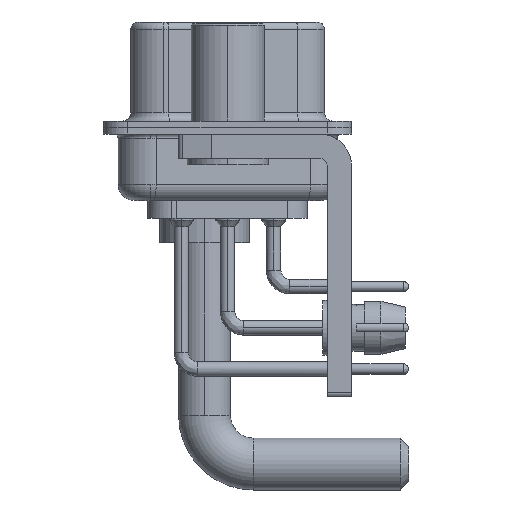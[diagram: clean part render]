
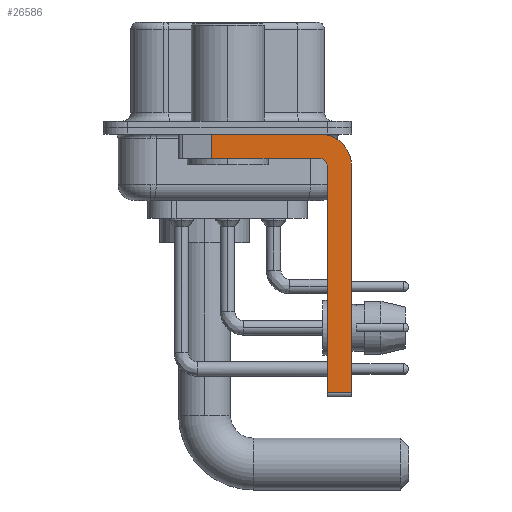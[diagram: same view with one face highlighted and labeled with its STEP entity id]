
A CAD part, left-side view. The second image highlights one B-rep face of the part: STEP entity #26586.
In plain terms, the highlighted planar face has unit normal (-1, 0, 0).
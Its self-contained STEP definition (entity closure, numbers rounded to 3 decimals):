
#164 = ORIENTED_EDGE ( 'NONE', *, *, #16579, .F. ) ;
#937 = CARTESIAN_POINT ( 'NONE',  ( -2.9, 0.978, -1.9 ) ) ;
#2447 = ORIENTED_EDGE ( 'NONE', *, *, #3373, .F. ) ;
#3217 = CARTESIAN_POINT ( 'NONE',  ( -2.9, -5.65, -2.4 ) ) ;
#3373 = EDGE_CURVE ( 'NONE', #6912, #23602, #33121, .T. ) ;
#3415 = EDGE_CURVE ( 'NONE', #27893, #8303, #26607, .T. ) ;
#3915 = AXIS2_PLACEMENT_3D ( 'NONE', #36404, #33342, #8636 ) ;
#4484 = VERTEX_POINT ( 'NONE', #37682 ) ;
#4507 = EDGE_CURVE ( 'NONE', #18690, #8303, #25046, .T. ) ;
#5152 = FACE_OUTER_BOUND ( 'NONE', #33756, .T. ) ;
#5398 = LINE ( 'NONE', #17841, #13800 ) ;
#5410 = AXIS2_PLACEMENT_3D ( 'NONE', #33012, #17060, #36479 ) ;
#5933 = AXIS2_PLACEMENT_3D ( 'NONE', #3217, #28167, #9552 ) ;
#6912 = VERTEX_POINT ( 'NONE', #35446 ) ;
#7973 = CARTESIAN_POINT ( 'NONE',  ( -2.9, -6.15, -16.35 ) ) ;
#8303 = VERTEX_POINT ( 'NONE', #12050 ) ;
#8636 = DIRECTION ( 'NONE',  ( 0., 0., -1. ) ) ;
#8646 = LINE ( 'NONE', #30895, #10267 ) ;
#9231 = ORIENTED_EDGE ( 'NONE', *, *, #22235, .F. ) ;
#9552 = DIRECTION ( 'NONE',  ( 0., 0., 1. ) ) ;
#10046 = EDGE_CURVE ( 'NONE', #30020, #6912, #37889, .T. ) ;
#10143 = ORIENTED_EDGE ( 'NONE', *, *, #3415, .T. ) ;
#10267 = VECTOR ( 'NONE', #33157, 1000. ) ;
#10851 = DIRECTION ( 'NONE',  ( 0., -1., 0. ) ) ;
#11998 = ORIENTED_EDGE ( 'NONE', *, *, #4507, .F. ) ;
#12050 = CARTESIAN_POINT ( 'NONE',  ( -2.9, -7.65, -16.35 ) ) ;
#12092 = EDGE_CURVE ( 'NONE', #27893, #30020, #5398, .T. ) ;
#12316 = CARTESIAN_POINT ( 'NONE',  ( -2.9, 0.978, -1.9 ) ) ;
#13800 = VECTOR ( 'NONE', #26881, 1000. ) ;
#13990 = LINE ( 'NONE', #937, #34609 ) ;
#16579 = EDGE_CURVE ( 'NONE', #4484, #18690, #20413, .T. ) ;
#16966 = DIRECTION ( 'NONE',  ( 0., 1., 0. ) ) ;
#17060 = DIRECTION ( 'NONE',  ( 1., 0., 0. ) ) ;
#17841 = CARTESIAN_POINT ( 'NONE',  ( -2.9, -6.15, -16.6 ) ) ;
#18450 = CARTESIAN_POINT ( 'NONE',  ( -2.9, 0.978, -0.4 ) ) ;
#18690 = VERTEX_POINT ( 'NONE', #37324 ) ;
#20413 = CIRCLE ( 'NONE', #5410, 2. ) ;
#20551 = VECTOR ( 'NONE', #10851, 1000. ) ;
#21968 = DIRECTION ( 'NONE',  ( 0., 0., -1. ) ) ;
#22235 = EDGE_CURVE ( 'NONE', #26379, #4484, #8646, .T. ) ;
#23130 = CARTESIAN_POINT ( 'NONE',  ( -2.9, -5.65, -1.9 ) ) ;
#23602 = VERTEX_POINT ( 'NONE', #12316 ) ;
#23972 = CARTESIAN_POINT ( 'NONE',  ( -2.9, -6.15, -2.4 ) ) ;
#25046 = LINE ( 'NONE', #34623, #28529 ) ;
#26379 = VERTEX_POINT ( 'NONE', #18450 ) ;
#26586 = ADVANCED_FACE ( 'NONE', ( #5152 ), #39665, .F. ) ;
#26607 = LINE ( 'NONE', #27222, #20551 ) ;
#26881 = DIRECTION ( 'NONE',  ( 0., 0., 1. ) ) ;
#27222 = CARTESIAN_POINT ( 'NONE',  ( -2.9, -5.65, -16.35 ) ) ;
#27275 = EDGE_CURVE ( 'NONE', #26379, #23602, #13990, .T. ) ;
#27893 = VERTEX_POINT ( 'NONE', #7973 ) ;
#28167 = DIRECTION ( 'NONE',  ( -1., 0., 0. ) ) ;
#28529 = VECTOR ( 'NONE', #21968, 1000. ) ;
#28938 = DIRECTION ( 'NONE',  ( 0., 0., -1. ) ) ;
#30020 = VERTEX_POINT ( 'NONE', #23972 ) ;
#30895 = CARTESIAN_POINT ( 'NONE',  ( -2.9, 3., -0.4 ) ) ;
#33012 = CARTESIAN_POINT ( 'NONE',  ( -2.9, -5.65, -2.4 ) ) ;
#33121 = LINE ( 'NONE', #23130, #38811 ) ;
#33157 = DIRECTION ( 'NONE',  ( 0., -1., 0. ) ) ;
#33342 = DIRECTION ( 'NONE',  ( 1., 0., 0. ) ) ;
#33756 = EDGE_LOOP ( 'NONE', ( #9231, #36742, #2447, #38156, #35592, #10143, #11998, #164 ) ) ;
#34609 = VECTOR ( 'NONE', #28938, 1000. ) ;
#34623 = CARTESIAN_POINT ( 'NONE',  ( -2.9, -7.65, -2.4 ) ) ;
#35446 = CARTESIAN_POINT ( 'NONE',  ( -2.9, -5.65, -1.9 ) ) ;
#35592 = ORIENTED_EDGE ( 'NONE', *, *, #12092, .F. ) ;
#36404 = CARTESIAN_POINT ( 'NONE',  ( -2.9, -5.65, -2.4 ) ) ;
#36479 = DIRECTION ( 'NONE',  ( 0., 0., -1. ) ) ;
#36742 = ORIENTED_EDGE ( 'NONE', *, *, #27275, .T. ) ;
#37324 = CARTESIAN_POINT ( 'NONE',  ( -2.9, -7.65, -2.4 ) ) ;
#37682 = CARTESIAN_POINT ( 'NONE',  ( -2.9, -5.65, -0.4 ) ) ;
#37889 = CIRCLE ( 'NONE', #5933, 0.5 ) ;
#38156 = ORIENTED_EDGE ( 'NONE', *, *, #10046, .F. ) ;
#38811 = VECTOR ( 'NONE', #16966, 1000. ) ;
#39665 = PLANE ( 'NONE',  #3915 ) ;
